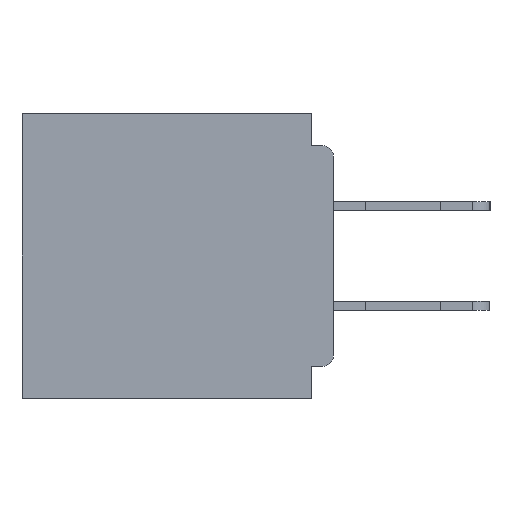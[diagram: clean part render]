
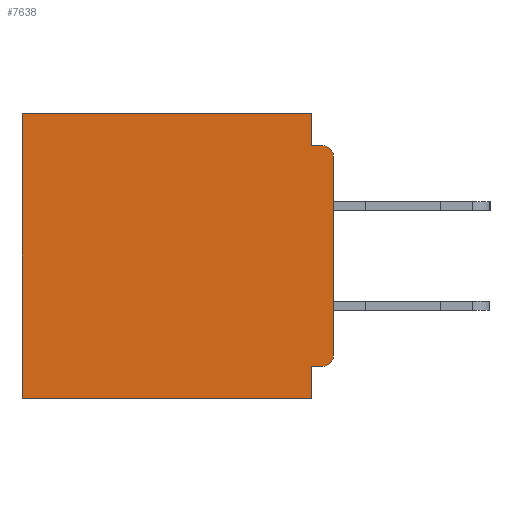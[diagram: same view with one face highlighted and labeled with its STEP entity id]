
A CAD part, left-side view. The second image highlights one B-rep face of the part: STEP entity #7638.
In plain terms, the highlighted planar face has unit normal (-1, 0, 0).
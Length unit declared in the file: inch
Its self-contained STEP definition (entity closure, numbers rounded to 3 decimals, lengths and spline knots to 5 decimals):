
#20 = ORIENTED_EDGE ( 'NONE', *, *, #9652, .F. ) ;
#26 = EDGE_CURVE ( 'NONE', #19170, #21914, #40629, .T. ) ;
#139 = DIRECTION ( 'NONE',  ( 0., 0., -1. ) ) ;
#181 = VECTOR ( 'NONE', #45131, 39.37008 ) ;
#1833 = VECTOR ( 'NONE', #56739, 39.37008 ) ;
#2042 = ORIENTED_EDGE ( 'NONE', *, *, #24062, .F. ) ;
#2064 = CARTESIAN_POINT ( 'NONE',  ( 0.3, 0.437, 0. ) ) ;
#2246 = ORIENTED_EDGE ( 'NONE', *, *, #20761, .F. ) ;
#3036 = CARTESIAN_POINT ( 'NONE',  ( 0.3, 0.437, -0.4 ) ) ;
#3350 = VECTOR ( 'NONE', #14859, 39.37008 ) ;
#5706 = CARTESIAN_POINT ( 'NONE',  ( 0.3, 0., -0.4 ) ) ;
#6216 = CARTESIAN_POINT ( 'NONE',  ( 0.3, 0.015, -0.06 ) ) ;
#6618 = VECTOR ( 'NONE', #23316, 39.37008 ) ;
#6963 = LINE ( 'NONE', #31282, #17573 ) ;
#7392 = ORIENTED_EDGE ( 'NONE', *, *, #46097, .F. ) ;
#7638 = ADVANCED_FACE ( 'NONE', ( #29320 ), #35829, .F. ) ;
#8035 = LINE ( 'NONE', #18825, #6618 ) ;
#8267 = DIRECTION ( 'NONE',  ( -1., 0., 0. ) ) ;
#9652 = EDGE_CURVE ( 'NONE', #53543, #42030, #34657, .T. ) ;
#9781 = CARTESIAN_POINT ( 'NONE',  ( 0.3, 0.015, -0.045 ) ) ;
#10684 = DIRECTION ( 'NONE',  ( 0., 0., -1. ) ) ;
#11302 = VECTOR ( 'NONE', #42619, 39.37008 ) ;
#14271 = VERTEX_POINT ( 'NONE', #49186 ) ;
#14859 = DIRECTION ( 'NONE',  ( 0., 1., 0. ) ) ;
#14960 = CARTESIAN_POINT ( 'NONE',  ( 0.3, 0.031, 0. ) ) ;
#15298 = LINE ( 'NONE', #46236, #3350 ) ;
#15817 = EDGE_CURVE ( 'NONE', #23133, #42260, #25771, .T. ) ;
#17397 = ORIENTED_EDGE ( 'NONE', *, *, #47143, .T. ) ;
#17458 = ORIENTED_EDGE ( 'NONE', *, *, #26, .F. ) ;
#17573 = VECTOR ( 'NONE', #44852, 39.37008 ) ;
#18825 = CARTESIAN_POINT ( 'NONE',  ( 0.3, 0., -0.045 ) ) ;
#18828 = ORIENTED_EDGE ( 'NONE', *, *, #41044, .F. ) ;
#19170 = VERTEX_POINT ( 'NONE', #44079 ) ;
#20761 = EDGE_CURVE ( 'NONE', #37491, #53543, #15298, .T. ) ;
#20791 = ORIENTED_EDGE ( 'NONE', *, *, #21247, .T. ) ;
#21247 = EDGE_CURVE ( 'NONE', #19170, #34372, #39105, .T. ) ;
#21286 = EDGE_LOOP ( 'NONE', ( #17458, #20791, #7392, #18828, #57334, #54939, #2042, #20, #2246, #17397 ) ) ;
#21914 = VERTEX_POINT ( 'NONE', #43035 ) ;
#23133 = VERTEX_POINT ( 'NONE', #2064 ) ;
#23316 = DIRECTION ( 'NONE',  ( 0., -1., 0. ) ) ;
#24062 = EDGE_CURVE ( 'NONE', #42030, #42260, #25521, .T. ) ;
#25521 = LINE ( 'NONE', #5706, #181 ) ;
#25771 = LINE ( 'NONE', #3036, #1833 ) ;
#27055 = DIRECTION ( 'NONE',  ( 1., 0., 0. ) ) ;
#29320 = FACE_OUTER_BOUND ( 'NONE', #21286, .T. ) ;
#29966 = AXIS2_PLACEMENT_3D ( 'NONE', #35092, #8267, #39655 ) ;
#30071 = VECTOR ( 'NONE', #47337, 39.37008 ) ;
#31282 = CARTESIAN_POINT ( 'NONE',  ( 0.3, 0.031, 0. ) ) ;
#33256 = VECTOR ( 'NONE', #56800, 39.37008 ) ;
#33730 = CARTESIAN_POINT ( 'NONE',  ( 0.3, 0., 0. ) ) ;
#33827 = CIRCLE ( 'NONE', #29966, 0.015 ) ;
#33947 = EDGE_CURVE ( 'NONE', #46848, #23133, #48540, .T. ) ;
#34372 = VERTEX_POINT ( 'NONE', #9781 ) ;
#34421 = AXIS2_PLACEMENT_3D ( 'NONE', #6216, #37565, #10684 ) ;
#34657 = LINE ( 'NONE', #52348, #33256 ) ;
#35092 = CARTESIAN_POINT ( 'NONE',  ( 0.3, 0.015, -0.34 ) ) ;
#35806 = CARTESIAN_POINT ( 'NONE',  ( 0.3, 0.031, -0.355 ) ) ;
#35829 = PLANE ( 'NONE',  #56035 ) ;
#37491 = VERTEX_POINT ( 'NONE', #40596 ) ;
#37565 = DIRECTION ( 'NONE',  ( -1., 0., 0. ) ) ;
#38003 = CARTESIAN_POINT ( 'NONE',  ( 0.3, 0.437, -0.4 ) ) ;
#39105 = CIRCLE ( 'NONE', #34421, 0.015 ) ;
#39655 = DIRECTION ( 'NONE',  ( 0., 0., -1. ) ) ;
#40394 = CARTESIAN_POINT ( 'NONE',  ( 0.3, 0., -0.4 ) ) ;
#40596 = CARTESIAN_POINT ( 'NONE',  ( 0.3, 0.015, -0.355 ) ) ;
#40629 = LINE ( 'NONE', #47419, #30071 ) ;
#41044 = EDGE_CURVE ( 'NONE', #46848, #14271, #6963, .T. ) ;
#42030 = VERTEX_POINT ( 'NONE', #54275 ) ;
#42260 = VERTEX_POINT ( 'NONE', #38003 ) ;
#42619 = DIRECTION ( 'NONE',  ( 0., 1., 0. ) ) ;
#43035 = CARTESIAN_POINT ( 'NONE',  ( 0.3, 0., -0.34 ) ) ;
#44079 = CARTESIAN_POINT ( 'NONE',  ( 0.3, 0., -0.06 ) ) ;
#44852 = DIRECTION ( 'NONE',  ( 0., 0., -1. ) ) ;
#45131 = DIRECTION ( 'NONE',  ( 0., 1., 0. ) ) ;
#46097 = EDGE_CURVE ( 'NONE', #14271, #34372, #8035, .T. ) ;
#46236 = CARTESIAN_POINT ( 'NONE',  ( 0.3, 0., -0.355 ) ) ;
#46848 = VERTEX_POINT ( 'NONE', #14960 ) ;
#47143 = EDGE_CURVE ( 'NONE', #37491, #21914, #33827, .T. ) ;
#47337 = DIRECTION ( 'NONE',  ( 0., 0., -1. ) ) ;
#47419 = CARTESIAN_POINT ( 'NONE',  ( 0.3, 0., -0.4 ) ) ;
#48540 = LINE ( 'NONE', #33730, #11302 ) ;
#49186 = CARTESIAN_POINT ( 'NONE',  ( 0.3, 0.031, -0.045 ) ) ;
#52348 = CARTESIAN_POINT ( 'NONE',  ( 0.3, 0.031, -0.4 ) ) ;
#53543 = VERTEX_POINT ( 'NONE', #35806 ) ;
#54275 = CARTESIAN_POINT ( 'NONE',  ( 0.3, 0.031, -0.4 ) ) ;
#54939 = ORIENTED_EDGE ( 'NONE', *, *, #15817, .T. ) ;
#56035 = AXIS2_PLACEMENT_3D ( 'NONE', #40394, #27055, #139 ) ;
#56739 = DIRECTION ( 'NONE',  ( 0., 0., -1. ) ) ;
#56800 = DIRECTION ( 'NONE',  ( 0., 0., -1. ) ) ;
#57334 = ORIENTED_EDGE ( 'NONE', *, *, #33947, .T. ) ;
